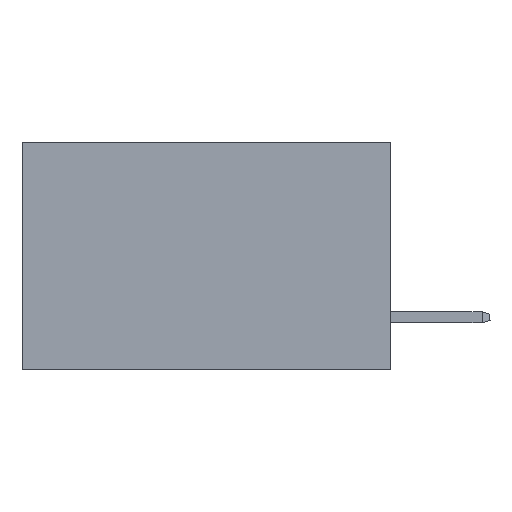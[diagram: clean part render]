
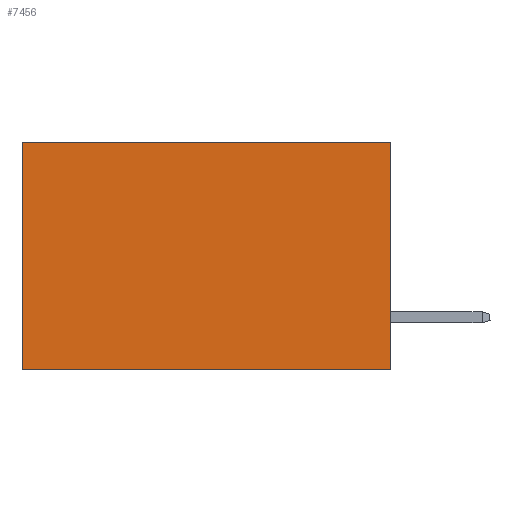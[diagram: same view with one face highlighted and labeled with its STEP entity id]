
A CAD part, left-side view. The second image highlights one B-rep face of the part: STEP entity #7456.
In plain terms, the highlighted planar face has unit normal (-1, 0, 0).
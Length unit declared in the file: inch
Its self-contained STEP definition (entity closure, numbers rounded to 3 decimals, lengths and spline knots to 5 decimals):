
#273 = DIRECTION ( 'NONE',  ( 0., 0., -1. ) ) ;
#1048 = ORIENTED_EDGE ( 'NONE', *, *, #19415, .F. ) ;
#1281 = AXIS2_PLACEMENT_3D ( 'NONE', #22856, #7486, #11400 ) ;
#1797 = LINE ( 'NONE', #18412, #4519 ) ;
#2208 = LINE ( 'NONE', #21818, #10456 ) ;
#3730 = EDGE_CURVE ( 'NONE', #13110, #4992, #2208, .T. ) ;
#4519 = VECTOR ( 'NONE', #24040, 39.37008 ) ;
#4667 = EDGE_LOOP ( 'NONE', ( #7142, #10086, #1048, #11044 ) ) ;
#4748 = DIRECTION ( 'NONE',  ( 0., 1., 0. ) ) ;
#4992 = VERTEX_POINT ( 'NONE', #21716 ) ;
#5953 = LINE ( 'NONE', #15611, #14859 ) ;
#7142 = ORIENTED_EDGE ( 'NONE', *, *, #14506, .T. ) ;
#7456 = ADVANCED_FACE ( 'NONE', ( #11459 ), #16946, .F. ) ;
#7486 = DIRECTION ( 'NONE',  ( 1., 0., 0. ) ) ;
#9041 = LINE ( 'NONE', #21503, #12570 ) ;
#10086 = ORIENTED_EDGE ( 'NONE', *, *, #17527, .F. ) ;
#10456 = VECTOR ( 'NONE', #4748, 39.37008 ) ;
#11044 = ORIENTED_EDGE ( 'NONE', *, *, #3730, .T. ) ;
#11400 = DIRECTION ( 'NONE',  ( 0., 0., -1. ) ) ;
#11459 = FACE_OUTER_BOUND ( 'NONE', #4667, .T. ) ;
#11970 = DIRECTION ( 'NONE',  ( 0., 1., 0. ) ) ;
#12570 = VECTOR ( 'NONE', #11970, 39.37008 ) ;
#13110 = VERTEX_POINT ( 'NONE', #15807 ) ;
#14506 = EDGE_CURVE ( 'NONE', #4992, #23489, #1797, .T. ) ;
#14859 = VECTOR ( 'NONE', #273, 39.37008 ) ;
#15611 = CARTESIAN_POINT ( 'NONE',  ( 0.2875, 0., 0. ) ) ;
#15807 = CARTESIAN_POINT ( 'NONE',  ( 0.2875, 0., 0. ) ) ;
#16445 = VERTEX_POINT ( 'NONE', #23957 ) ;
#16946 = PLANE ( 'NONE',  #1281 ) ;
#17527 = EDGE_CURVE ( 'NONE', #16445, #23489, #9041, .T. ) ;
#18412 = CARTESIAN_POINT ( 'NONE',  ( 0.2875, 0.6, 0. ) ) ;
#19415 = EDGE_CURVE ( 'NONE', #13110, #16445, #5953, .T. ) ;
#19720 = CARTESIAN_POINT ( 'NONE',  ( 0.2875, 0.6, -0.37 ) ) ;
#21503 = CARTESIAN_POINT ( 'NONE',  ( 0.2875, 0., -0.37 ) ) ;
#21716 = CARTESIAN_POINT ( 'NONE',  ( 0.2875, 0.6, 0. ) ) ;
#21818 = CARTESIAN_POINT ( 'NONE',  ( 0.2875, 0., 0. ) ) ;
#22856 = CARTESIAN_POINT ( 'NONE',  ( 0.2875, 0., 0. ) ) ;
#23489 = VERTEX_POINT ( 'NONE', #19720 ) ;
#23957 = CARTESIAN_POINT ( 'NONE',  ( 0.2875, 0., -0.37 ) ) ;
#24040 = DIRECTION ( 'NONE',  ( 0., 0., -1. ) ) ;
